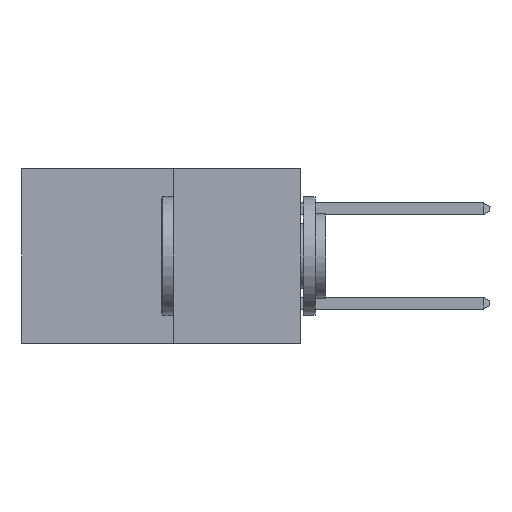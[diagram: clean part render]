
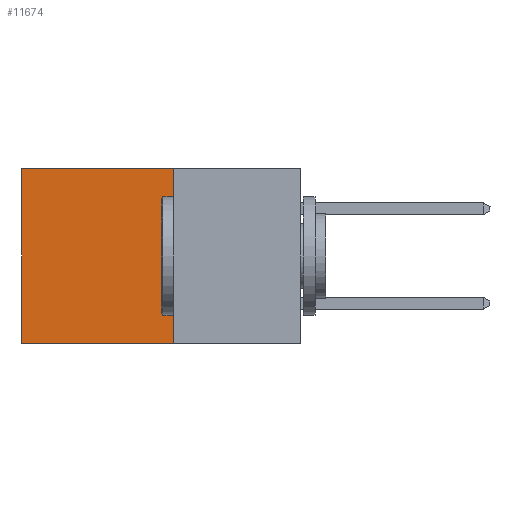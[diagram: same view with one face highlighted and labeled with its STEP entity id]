
A CAD part, left-side view. The second image highlights one B-rep face of the part: STEP entity #11674.
In plain terms, the highlighted planar face has unit normal (-1, 0, 0).
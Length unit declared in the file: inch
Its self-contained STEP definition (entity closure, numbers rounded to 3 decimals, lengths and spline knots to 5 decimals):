
#372 = LINE ( 'NONE', #13128, #6789 ) ;
#385 = VERTEX_POINT ( 'NONE', #10055 ) ;
#1274 = VERTEX_POINT ( 'NONE', #7510 ) ;
#2168 = VECTOR ( 'NONE', #4826, 39.37008 ) ;
#2548 = PLANE ( 'NONE',  #9793 ) ;
#2623 = FACE_OUTER_BOUND ( 'NONE', #8183, .T. ) ;
#3847 = CARTESIAN_POINT ( 'NONE',  ( 0.277, 0.27, -0.37 ) ) ;
#3894 = ORIENTED_EDGE ( 'NONE', *, *, #5972, .T. ) ;
#3950 = VERTEX_POINT ( 'NONE', #15777 ) ;
#4826 = DIRECTION ( 'NONE',  ( 0., 1., 0. ) ) ;
#5103 = CARTESIAN_POINT ( 'NONE',  ( 0.277, 0.27, 0. ) ) ;
#5147 = DIRECTION ( 'NONE',  ( 0., 0., -1. ) ) ;
#5972 = EDGE_CURVE ( 'NONE', #385, #13787, #12248, .T. ) ;
#6337 = ORIENTED_EDGE ( 'NONE', *, *, #14686, .F. ) ;
#6789 = VECTOR ( 'NONE', #11888, 39.37008 ) ;
#7510 = CARTESIAN_POINT ( 'NONE',  ( 0.277, 0.27, -0.37 ) ) ;
#8183 = EDGE_LOOP ( 'NONE', ( #15262, #13710, #6337, #3894 ) ) ;
#8212 = VECTOR ( 'NONE', #13290, 39.37008 ) ;
#8703 = DIRECTION ( 'NONE',  ( 0., 1., 0. ) ) ;
#9793 = AXIS2_PLACEMENT_3D ( 'NONE', #3847, #12633, #5147 ) ;
#10055 = CARTESIAN_POINT ( 'NONE',  ( 0.277, 0.27, 0. ) ) ;
#11186 = CARTESIAN_POINT ( 'NONE',  ( 0.277, 0.27, -0.37 ) ) ;
#11674 = ADVANCED_FACE ( 'NONE', ( #2623 ), #2548, .F. ) ;
#11683 = CARTESIAN_POINT ( 'NONE',  ( 0.277, 0.59, 0. ) ) ;
#11888 = DIRECTION ( 'NONE',  ( 0., 0., -1. ) ) ;
#12046 = CARTESIAN_POINT ( 'NONE',  ( 0.277, 0.27, -0.37 ) ) ;
#12065 = VECTOR ( 'NONE', #8703, 39.37008 ) ;
#12248 = LINE ( 'NONE', #5103, #2168 ) ;
#12633 = DIRECTION ( 'NONE',  ( 1., 0., 0. ) ) ;
#12858 = EDGE_CURVE ( 'NONE', #1274, #3950, #15349, .T. ) ;
#13128 = CARTESIAN_POINT ( 'NONE',  ( 0.277, 0.59, -0.37 ) ) ;
#13290 = DIRECTION ( 'NONE',  ( 0., 0., -1. ) ) ;
#13710 = ORIENTED_EDGE ( 'NONE', *, *, #12858, .F. ) ;
#13787 = VERTEX_POINT ( 'NONE', #11683 ) ;
#14686 = EDGE_CURVE ( 'NONE', #385, #1274, #14764, .T. ) ;
#14764 = LINE ( 'NONE', #12046, #8212 ) ;
#15262 = ORIENTED_EDGE ( 'NONE', *, *, #16119, .T. ) ;
#15349 = LINE ( 'NONE', #11186, #12065 ) ;
#15777 = CARTESIAN_POINT ( 'NONE',  ( 0.277, 0.59, -0.37 ) ) ;
#16119 = EDGE_CURVE ( 'NONE', #13787, #3950, #372, .T. ) ;
